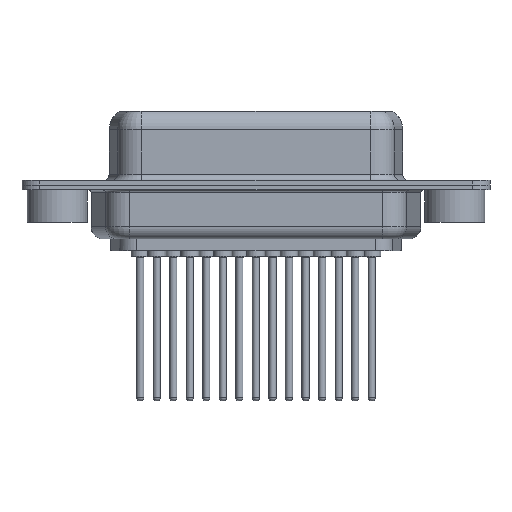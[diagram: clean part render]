
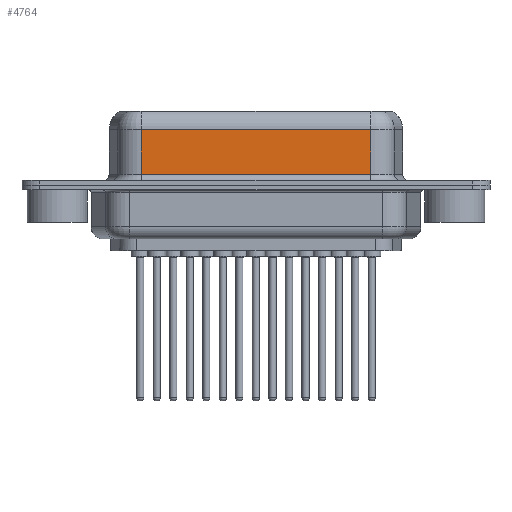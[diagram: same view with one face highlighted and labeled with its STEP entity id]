
A CAD part, front view. The second image highlights one B-rep face of the part: STEP entity #4764.
In plain terms, the highlighted planar face has unit normal (0, -1, 0).
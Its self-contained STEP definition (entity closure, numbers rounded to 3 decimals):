
#209 = CARTESIAN_POINT ( 'NONE',  ( 7.038, -3.95, 4.65 ) ) ;
#394 = CARTESIAN_POINT ( 'NONE',  ( 26.262, -3.95, 4.65 ) ) ;
#437 = CARTESIAN_POINT ( 'NONE',  ( 26.262, -3.95, 6.4 ) ) ;
#484 = VECTOR ( 'NONE', #12621, 1000. ) ;
#493 = DIRECTION ( 'NONE',  ( 0., 1., 0. ) ) ;
#2024 = FACE_OUTER_BOUND ( 'NONE', #13485, .T. ) ;
#2833 = CARTESIAN_POINT ( 'NONE',  ( 26.262, -3.95, 0.9 ) ) ;
#2874 = ORIENTED_EDGE ( 'NONE', *, *, #2972, .T. ) ;
#2972 = EDGE_CURVE ( 'NONE', #5211, #14898, #5119, .T. ) ;
#3028 = CARTESIAN_POINT ( 'NONE',  ( 26.262, -3.95, 4.65 ) ) ;
#4113 = CARTESIAN_POINT ( 'NONE',  ( 7.038, -3.95, 0.9 ) ) ;
#4270 = EDGE_CURVE ( 'NONE', #6273, #13859, #16986, .T. ) ;
#4578 = CARTESIAN_POINT ( 'NONE',  ( 26.262, -3.95, 6.4 ) ) ;
#4764 = ADVANCED_FACE ( 'NONE', ( #2024 ), #7204, .F. ) ;
#5021 = EDGE_CURVE ( 'NONE', #14898, #13859, #10803, .T. ) ;
#5119 = LINE ( 'NONE', #6211, #8030 ) ;
#5211 = VERTEX_POINT ( 'NONE', #209 ) ;
#6211 = CARTESIAN_POINT ( 'NONE',  ( 7.038, -3.95, 6.4 ) ) ;
#6273 = VERTEX_POINT ( 'NONE', #3028 ) ;
#6283 = ORIENTED_EDGE ( 'NONE', *, *, #5021, .T. ) ;
#6714 = AXIS2_PLACEMENT_3D ( 'NONE', #4578, #493, #12742 ) ;
#7149 = EDGE_CURVE ( 'NONE', #6273, #5211, #15588, .T. ) ;
#7204 = PLANE ( 'NONE',  #6714 ) ;
#8030 = VECTOR ( 'NONE', #10639, 1000. ) ;
#8763 = DIRECTION ( 'NONE',  ( 0., 0., -1. ) ) ;
#9241 = VECTOR ( 'NONE', #8763, 1000. ) ;
#10639 = DIRECTION ( 'NONE',  ( 0., 0., -1. ) ) ;
#10803 = LINE ( 'NONE', #2833, #484 ) ;
#12621 = DIRECTION ( 'NONE',  ( 1., 0., 0. ) ) ;
#12742 = DIRECTION ( 'NONE',  ( -1., 0., 0. ) ) ;
#12808 = DIRECTION ( 'NONE',  ( -1., 0., 0. ) ) ;
#12873 = VECTOR ( 'NONE', #12808, 1000. ) ;
#13485 = EDGE_LOOP ( 'NONE', ( #17334, #17499, #2874, #6283 ) ) ;
#13859 = VERTEX_POINT ( 'NONE', #14314 ) ;
#14314 = CARTESIAN_POINT ( 'NONE',  ( 26.262, -3.95, 0.9 ) ) ;
#14898 = VERTEX_POINT ( 'NONE', #4113 ) ;
#15588 = LINE ( 'NONE', #394, #12873 ) ;
#16986 = LINE ( 'NONE', #437, #9241 ) ;
#17334 = ORIENTED_EDGE ( 'NONE', *, *, #4270, .F. ) ;
#17499 = ORIENTED_EDGE ( 'NONE', *, *, #7149, .T. ) ;
